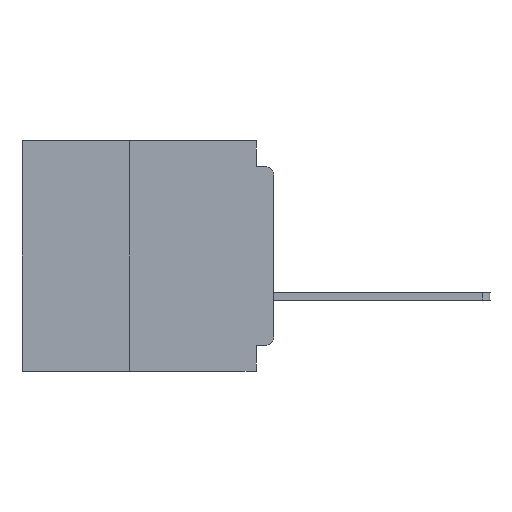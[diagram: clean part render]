
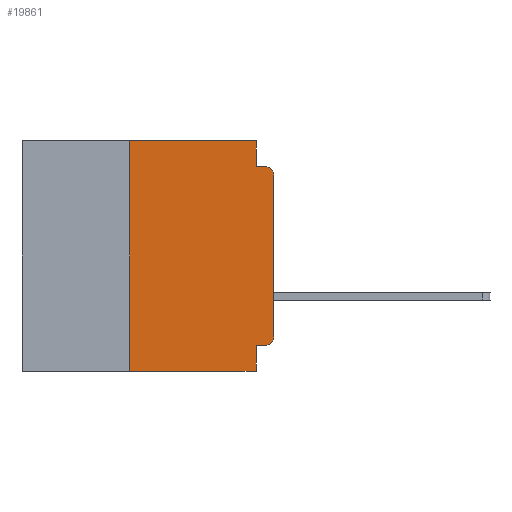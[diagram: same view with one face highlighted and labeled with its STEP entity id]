
A CAD part, left-side view. The second image highlights one B-rep face of the part: STEP entity #19861.
In plain terms, the highlighted planar face has unit normal (-1, 0, 0).
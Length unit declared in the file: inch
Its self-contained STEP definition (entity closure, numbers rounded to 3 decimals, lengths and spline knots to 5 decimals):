
#689 = DIRECTION ( 'NONE',  ( 0., 0., -1. ) ) ;
#1126 = CARTESIAN_POINT ( 'NONE',  ( 0., 0.031, -0.045 ) ) ;
#4086 = LINE ( 'NONE', #23231, #29432 ) ;
#4375 = DIRECTION ( 'NONE',  ( -1., 0., 0. ) ) ;
#4965 = VERTEX_POINT ( 'NONE', #48985 ) ;
#5055 = VECTOR ( 'NONE', #53289, 39.37008 ) ;
#5306 = EDGE_CURVE ( 'NONE', #58984, #36421, #60138, .T. ) ;
#5842 = CARTESIAN_POINT ( 'NONE',  ( 0., 0.031, -0.4 ) ) ;
#6155 = CARTESIAN_POINT ( 'NONE',  ( 0., 0.015, -0.355 ) ) ;
#6419 = ORIENTED_EDGE ( 'NONE', *, *, #63145, .F. ) ;
#6906 = DIRECTION ( 'NONE',  ( -1., 0., 0. ) ) ;
#7008 = ORIENTED_EDGE ( 'NONE', *, *, #59586, .T. ) ;
#8260 = DIRECTION ( 'NONE',  ( 0., 0., -1. ) ) ;
#9636 = LINE ( 'NONE', #27534, #61807 ) ;
#10010 = CARTESIAN_POINT ( 'NONE',  ( 0., 0.25, 0. ) ) ;
#11246 = CIRCLE ( 'NONE', #56033, 0.015 ) ;
#11917 = EDGE_LOOP ( 'NONE', ( #55598, #33390, #17952, #6419, #35482, #50834, #38735, #23619, #23273, #7008 ) ) ;
#11954 = CARTESIAN_POINT ( 'NONE',  ( 0., 0.031, 0. ) ) ;
#12920 = PLANE ( 'NONE',  #45232 ) ;
#13164 = VECTOR ( 'NONE', #18567, 39.37008 ) ;
#14020 = DIRECTION ( 'NONE',  ( 0., 0., 1. ) ) ;
#15989 = EDGE_CURVE ( 'NONE', #44883, #49345, #9636, .T. ) ;
#16215 = CARTESIAN_POINT ( 'NONE',  ( 0., 0.437, 0. ) ) ;
#16671 = EDGE_CURVE ( 'NONE', #49229, #40047, #4086, .T. ) ;
#17952 = ORIENTED_EDGE ( 'NONE', *, *, #15989, .F. ) ;
#18567 = DIRECTION ( 'NONE',  ( 0., 1., 0. ) ) ;
#19861 = ADVANCED_FACE ( 'NONE', ( #44796 ), #12920, .F. ) ;
#21298 = DIRECTION ( 'NONE',  ( 0., -1., 0. ) ) ;
#21966 = EDGE_CURVE ( 'NONE', #61285, #40047, #47655, .T. ) ;
#22300 = VECTOR ( 'NONE', #689, 39.37008 ) ;
#22627 = AXIS2_PLACEMENT_3D ( 'NONE', #34729, #4375, #39797 ) ;
#23231 = CARTESIAN_POINT ( 'NONE',  ( 0., 0.437, -0.4 ) ) ;
#23273 = ORIENTED_EDGE ( 'NONE', *, *, #28716, .F. ) ;
#23619 = ORIENTED_EDGE ( 'NONE', *, *, #21966, .F. ) ;
#23890 = LINE ( 'NONE', #61300, #22300 ) ;
#24622 = CARTESIAN_POINT ( 'NONE',  ( 0., 0.031, -0.355 ) ) ;
#24683 = CARTESIAN_POINT ( 'NONE',  ( 0., 0.015, -0.045 ) ) ;
#27534 = CARTESIAN_POINT ( 'NONE',  ( 0., 0., -0.045 ) ) ;
#28369 = CARTESIAN_POINT ( 'NONE',  ( 0., 0.437, 0. ) ) ;
#28716 = EDGE_CURVE ( 'NONE', #36333, #61285, #40056, .T. ) ;
#29432 = VECTOR ( 'NONE', #38535, 39.37008 ) ;
#29500 = VECTOR ( 'NONE', #14020, 39.37008 ) ;
#31047 = CARTESIAN_POINT ( 'NONE',  ( 0., 0.031, -0.4 ) ) ;
#33007 = CARTESIAN_POINT ( 'NONE',  ( 0., 0., 0. ) ) ;
#33390 = ORIENTED_EDGE ( 'NONE', *, *, #48168, .T. ) ;
#34729 = CARTESIAN_POINT ( 'NONE',  ( 0., 0.015, -0.34 ) ) ;
#35482 = ORIENTED_EDGE ( 'NONE', *, *, #5306, .F. ) ;
#36333 = VERTEX_POINT ( 'NONE', #6155 ) ;
#36421 = VERTEX_POINT ( 'NONE', #11954 ) ;
#37243 = CARTESIAN_POINT ( 'NONE',  ( 0., 0.015, -0.06 ) ) ;
#37755 = DIRECTION ( 'NONE',  ( 0., -1., 0. ) ) ;
#38535 = DIRECTION ( 'NONE',  ( 0., -1., 0. ) ) ;
#38567 = DIRECTION ( 'NONE',  ( 1., 0., 0. ) ) ;
#38735 = ORIENTED_EDGE ( 'NONE', *, *, #16671, .T. ) ;
#39797 = DIRECTION ( 'NONE',  ( 0., 0., -1. ) ) ;
#40047 = VERTEX_POINT ( 'NONE', #5842 ) ;
#40056 = LINE ( 'NONE', #59061, #13164 ) ;
#42300 = DIRECTION ( 'NONE',  ( 0., 0., -1. ) ) ;
#44344 = CARTESIAN_POINT ( 'NONE',  ( 0., 0.25, -0.4 ) ) ;
#44796 = FACE_OUTER_BOUND ( 'NONE', #11917, .T. ) ;
#44883 = VERTEX_POINT ( 'NONE', #1126 ) ;
#45232 = AXIS2_PLACEMENT_3D ( 'NONE', #28369, #38567, #8260 ) ;
#45414 = LINE ( 'NONE', #33007, #5055 ) ;
#46272 = DIRECTION ( 'NONE',  ( 0., 0., -1. ) ) ;
#46716 = VECTOR ( 'NONE', #21298, 39.37008 ) ;
#47655 = LINE ( 'NONE', #31047, #59498 ) ;
#48168 = EDGE_CURVE ( 'NONE', #4965, #49345, #11246, .T. ) ;
#48985 = CARTESIAN_POINT ( 'NONE',  ( 0., 0., -0.06 ) ) ;
#49229 = VERTEX_POINT ( 'NONE', #55615 ) ;
#49345 = VERTEX_POINT ( 'NONE', #24683 ) ;
#50834 = ORIENTED_EDGE ( 'NONE', *, *, #62908, .F. ) ;
#53234 = LINE ( 'NONE', #44344, #29500 ) ;
#53289 = DIRECTION ( 'NONE',  ( 0., 0., 1. ) ) ;
#55598 = ORIENTED_EDGE ( 'NONE', *, *, #62170, .T. ) ;
#55615 = CARTESIAN_POINT ( 'NONE',  ( 0., 0.25, -0.4 ) ) ;
#56033 = AXIS2_PLACEMENT_3D ( 'NONE', #37243, #6906, #42300 ) ;
#58984 = VERTEX_POINT ( 'NONE', #10010 ) ;
#59061 = CARTESIAN_POINT ( 'NONE',  ( 0., 0., -0.355 ) ) ;
#59498 = VECTOR ( 'NONE', #46272, 39.37008 ) ;
#59586 = EDGE_CURVE ( 'NONE', #36333, #63259, #62485, .T. ) ;
#60138 = LINE ( 'NONE', #16215, #46716 ) ;
#61285 = VERTEX_POINT ( 'NONE', #24622 ) ;
#61300 = CARTESIAN_POINT ( 'NONE',  ( 0., 0.031, 0. ) ) ;
#61807 = VECTOR ( 'NONE', #37755, 39.37008 ) ;
#62170 = EDGE_CURVE ( 'NONE', #63259, #4965, #45414, .T. ) ;
#62485 = CIRCLE ( 'NONE', #22627, 0.015 ) ;
#62591 = CARTESIAN_POINT ( 'NONE',  ( 0., 0., -0.34 ) ) ;
#62908 = EDGE_CURVE ( 'NONE', #49229, #58984, #53234, .T. ) ;
#63145 = EDGE_CURVE ( 'NONE', #36421, #44883, #23890, .T. ) ;
#63259 = VERTEX_POINT ( 'NONE', #62591 ) ;
